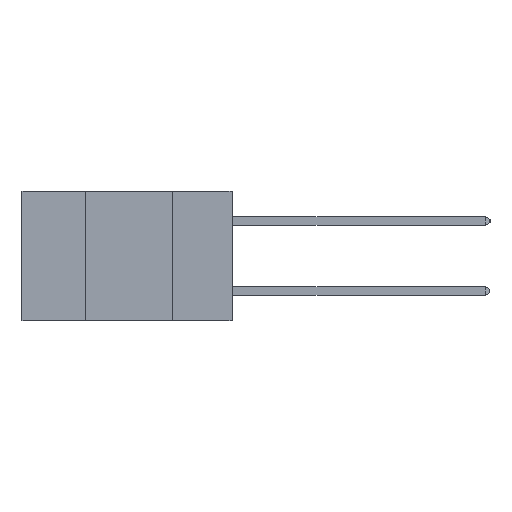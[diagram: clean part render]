
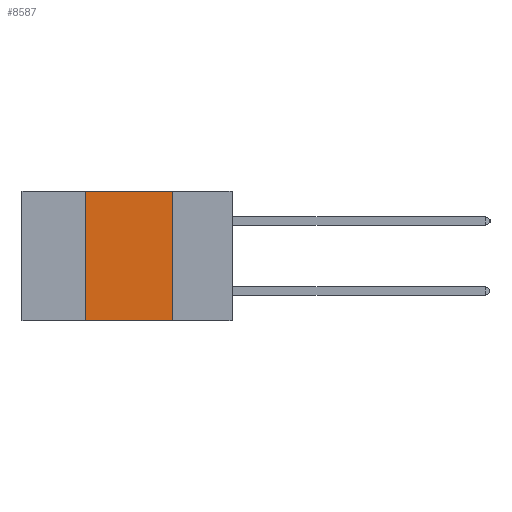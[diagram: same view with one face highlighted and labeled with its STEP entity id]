
A CAD part, left-side view. The second image highlights one B-rep face of the part: STEP entity #8587.
In plain terms, the highlighted planar face has unit normal (-1, 0, 0).
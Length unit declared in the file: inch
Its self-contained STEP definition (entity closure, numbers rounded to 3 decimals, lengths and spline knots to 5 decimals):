
#2854 = CARTESIAN_POINT ( 'NONE',  ( 0., 0.17, 0. ) ) ;
#2911 = ORIENTED_EDGE ( 'NONE', *, *, #8674, .F. ) ;
#3804 = LINE ( 'NONE', #9342, #9890 ) ;
#4122 = CARTESIAN_POINT ( 'NONE',  ( 0., 0.6, -0.37 ) ) ;
#4555 = ORIENTED_EDGE ( 'NONE', *, *, #4909, .F. ) ;
#4777 = CARTESIAN_POINT ( 'NONE',  ( 0., 0.17, -0.37 ) ) ;
#4909 = EDGE_CURVE ( 'NONE', #14776, #7588, #3804, .T. ) ;
#5815 = VECTOR ( 'NONE', #9186, 39.37008 ) ;
#5902 = DIRECTION ( 'NONE',  ( 0., 0., 1. ) ) ;
#6385 = ORIENTED_EDGE ( 'NONE', *, *, #10831, .F. ) ;
#6594 = VECTOR ( 'NONE', #7469, 39.37008 ) ;
#7077 = CARTESIAN_POINT ( 'NONE',  ( 0., 0.42, -0.37 ) ) ;
#7469 = DIRECTION ( 'NONE',  ( 0., 0., -1. ) ) ;
#7588 = VERTEX_POINT ( 'NONE', #13254 ) ;
#8167 = CARTESIAN_POINT ( 'NONE',  ( 0., 0.17, 0. ) ) ;
#8446 = CARTESIAN_POINT ( 'NONE',  ( 0., 0.6, 0. ) ) ;
#8587 = ADVANCED_FACE ( 'NONE', ( #13783 ), #9629, .F. ) ;
#8674 = EDGE_CURVE ( 'NONE', #11731, #11709, #12469, .T. ) ;
#9186 = DIRECTION ( 'NONE',  ( 0., -1., 0. ) ) ;
#9342 = CARTESIAN_POINT ( 'NONE',  ( 0., 0.42, 0. ) ) ;
#9629 = PLANE ( 'NONE',  #10585 ) ;
#9890 = VECTOR ( 'NONE', #5902, 39.37008 ) ;
#10585 = AXIS2_PLACEMENT_3D ( 'NONE', #8446, #13860, #10739 ) ;
#10739 = DIRECTION ( 'NONE',  ( 0., 0., -1. ) ) ;
#10831 = EDGE_CURVE ( 'NONE', #7588, #11731, #11818, .T. ) ;
#10923 = DIRECTION ( 'NONE',  ( 0., -1., 0. ) ) ;
#11246 = EDGE_CURVE ( 'NONE', #14776, #11709, #13406, .T. ) ;
#11401 = ORIENTED_EDGE ( 'NONE', *, *, #11246, .T. ) ;
#11709 = VERTEX_POINT ( 'NONE', #4777 ) ;
#11731 = VERTEX_POINT ( 'NONE', #8167 ) ;
#11803 = EDGE_LOOP ( 'NONE', ( #2911, #6385, #4555, #11401 ) ) ;
#11818 = LINE ( 'NONE', #13475, #5815 ) ;
#12469 = LINE ( 'NONE', #2854, #6594 ) ;
#13087 = VECTOR ( 'NONE', #10923, 39.37008 ) ;
#13254 = CARTESIAN_POINT ( 'NONE',  ( 0., 0.42, 0. ) ) ;
#13406 = LINE ( 'NONE', #4122, #13087 ) ;
#13475 = CARTESIAN_POINT ( 'NONE',  ( 0., 0.6, 0. ) ) ;
#13783 = FACE_OUTER_BOUND ( 'NONE', #11803, .T. ) ;
#13860 = DIRECTION ( 'NONE',  ( 1., 0., 0. ) ) ;
#14776 = VERTEX_POINT ( 'NONE', #7077 ) ;
